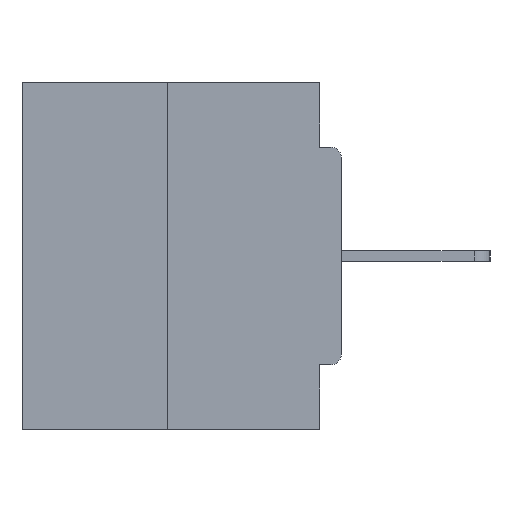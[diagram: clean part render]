
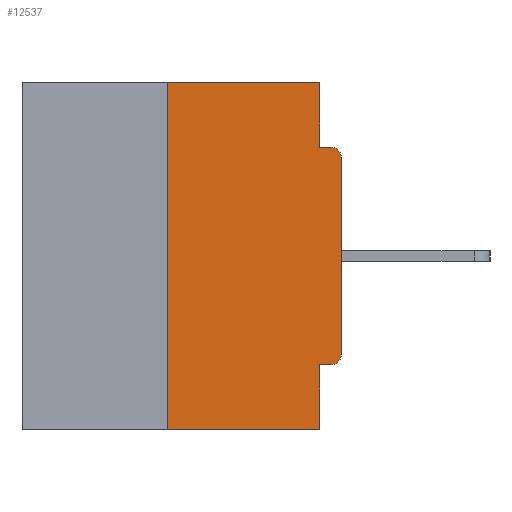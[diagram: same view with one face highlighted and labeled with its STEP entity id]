
A CAD part, left-side view. The second image highlights one B-rep face of the part: STEP entity #12537.
In plain terms, the highlighted planar face has unit normal (-1, 0, 0).
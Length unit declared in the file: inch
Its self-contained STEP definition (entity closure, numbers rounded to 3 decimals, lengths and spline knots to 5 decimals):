
#503 = DIRECTION ( 'NONE',  ( 0., 0., -1. ) ) ;
#929 = ORIENTED_EDGE ( 'NONE', *, *, #15177, .T. ) ;
#1581 = CARTESIAN_POINT ( 'NONE',  ( 0., 0.015, -0.4065 ) ) ;
#2330 = PLANE ( 'NONE',  #23668 ) ;
#2412 = VERTEX_POINT ( 'NONE', #6852 ) ;
#2626 = FACE_OUTER_BOUND ( 'NONE', #9411, .T. ) ;
#2676 = DIRECTION ( 'NONE',  ( 0., -1., 0. ) ) ;
#3253 = VECTOR ( 'NONE', #3336, 39.37008 ) ;
#3336 = DIRECTION ( 'NONE',  ( 0., 0., 1. ) ) ;
#3755 = DIRECTION ( 'NONE',  ( 0., 1., 0. ) ) ;
#4030 = LINE ( 'NONE', #31475, #20502 ) ;
#4177 = CARTESIAN_POINT ( 'NONE',  ( 0., 0.031, -0.5 ) ) ;
#4433 = LINE ( 'NONE', #6392, #27638 ) ;
#5618 = CARTESIAN_POINT ( 'NONE',  ( 0., 0.015, -0.3915 ) ) ;
#5665 = VERTEX_POINT ( 'NONE', #16105 ) ;
#6120 = LINE ( 'NONE', #13108, #3253 ) ;
#6241 = ORIENTED_EDGE ( 'NONE', *, *, #26397, .F. ) ;
#6304 = CARTESIAN_POINT ( 'NONE',  ( 0., 0.25, -0.5 ) ) ;
#6392 = CARTESIAN_POINT ( 'NONE',  ( 0., 0.25, 0. ) ) ;
#6852 = CARTESIAN_POINT ( 'NONE',  ( 0., 0.25, 0. ) ) ;
#7880 = VERTEX_POINT ( 'NONE', #9330 ) ;
#8070 = CARTESIAN_POINT ( 'NONE',  ( 0., 0., -0.4065 ) ) ;
#8222 = ORIENTED_EDGE ( 'NONE', *, *, #12829, .F. ) ;
#8256 = CARTESIAN_POINT ( 'NONE',  ( 0., 0.031, -0.0935 ) ) ;
#8479 = DIRECTION ( 'NONE',  ( 0., -1., 0. ) ) ;
#9048 = CARTESIAN_POINT ( 'NONE',  ( 0., 0.015, -0.1085 ) ) ;
#9330 = CARTESIAN_POINT ( 'NONE',  ( 0., 0.031, -0.4065 ) ) ;
#9411 = EDGE_LOOP ( 'NONE', ( #23773, #20358, #26169, #8222, #23984, #16713, #929, #14431, #6241, #16101 ) ) ;
#9448 = VERTEX_POINT ( 'NONE', #8256 ) ;
#9964 = EDGE_CURVE ( 'NONE', #26094, #10788, #29596, .T. ) ;
#10181 = DIRECTION ( 'NONE',  ( -1., 0., 0. ) ) ;
#10189 = LINE ( 'NONE', #24910, #29163 ) ;
#10788 = VERTEX_POINT ( 'NONE', #4177 ) ;
#11238 = EDGE_CURVE ( 'NONE', #30255, #18971, #11593, .T. ) ;
#11593 = CIRCLE ( 'NONE', #17828, 0.015 ) ;
#11639 = DIRECTION ( 'NONE',  ( 0., -1., 0. ) ) ;
#12537 = ADVANCED_FACE ( 'NONE', ( #2626 ), #2330, .F. ) ;
#12764 = CARTESIAN_POINT ( 'NONE',  ( 0., 0.031, 0. ) ) ;
#12829 = EDGE_CURVE ( 'NONE', #7880, #10788, #31689, .T. ) ;
#13108 = CARTESIAN_POINT ( 'NONE',  ( 0., 0., 0. ) ) ;
#13932 = EDGE_CURVE ( 'NONE', #21062, #7880, #16162, .T. ) ;
#14431 = ORIENTED_EDGE ( 'NONE', *, *, #11238, .T. ) ;
#15177 = EDGE_CURVE ( 'NONE', #5665, #30255, #6120, .T. ) ;
#15244 = VECTOR ( 'NONE', #23862, 39.37008 ) ;
#15352 = VECTOR ( 'NONE', #8479, 39.37008 ) ;
#15406 = CARTESIAN_POINT ( 'NONE',  ( 0., 0., -0.1085 ) ) ;
#15830 = LINE ( 'NONE', #23199, #15352 ) ;
#16101 = ORIENTED_EDGE ( 'NONE', *, *, #21096, .F. ) ;
#16105 = CARTESIAN_POINT ( 'NONE',  ( 0., 0., -0.3915 ) ) ;
#16162 = LINE ( 'NONE', #8070, #16819 ) ;
#16713 = ORIENTED_EDGE ( 'NONE', *, *, #30251, .T. ) ;
#16736 = DIRECTION ( 'NONE',  ( 0., 0., -1. ) ) ;
#16819 = VECTOR ( 'NONE', #3755, 39.37008 ) ;
#17487 = DIRECTION ( 'NONE',  ( 1., 0., 0. ) ) ;
#17828 = AXIS2_PLACEMENT_3D ( 'NONE', #9048, #22105, #26863 ) ;
#18017 = DIRECTION ( 'NONE',  ( 0., 0., -1. ) ) ;
#18971 = VERTEX_POINT ( 'NONE', #28110 ) ;
#19381 = AXIS2_PLACEMENT_3D ( 'NONE', #5618, #10181, #18017 ) ;
#20358 = ORIENTED_EDGE ( 'NONE', *, *, #27040, .F. ) ;
#20502 = VECTOR ( 'NONE', #16736, 39.37008 ) ;
#21062 = VERTEX_POINT ( 'NONE', #1581 ) ;
#21096 = EDGE_CURVE ( 'NONE', #21788, #9448, #4030, .T. ) ;
#21788 = VERTEX_POINT ( 'NONE', #12764 ) ;
#21997 = CIRCLE ( 'NONE', #19381, 0.015 ) ;
#22105 = DIRECTION ( 'NONE',  ( -1., 0., 0. ) ) ;
#22332 = EDGE_CURVE ( 'NONE', #2412, #21788, #15830, .T. ) ;
#23199 = CARTESIAN_POINT ( 'NONE',  ( 0., 0.46, 0. ) ) ;
#23668 = AXIS2_PLACEMENT_3D ( 'NONE', #27617, #17487, #503 ) ;
#23773 = ORIENTED_EDGE ( 'NONE', *, *, #22332, .F. ) ;
#23862 = DIRECTION ( 'NONE',  ( 0., 0., -1. ) ) ;
#23984 = ORIENTED_EDGE ( 'NONE', *, *, #13932, .F. ) ;
#24233 = CARTESIAN_POINT ( 'NONE',  ( 0., 0.46, -0.5 ) ) ;
#24910 = CARTESIAN_POINT ( 'NONE',  ( 0., 0., -0.0935 ) ) ;
#26094 = VERTEX_POINT ( 'NONE', #6304 ) ;
#26169 = ORIENTED_EDGE ( 'NONE', *, *, #9964, .T. ) ;
#26397 = EDGE_CURVE ( 'NONE', #9448, #18971, #10189, .T. ) ;
#26863 = DIRECTION ( 'NONE',  ( 0., 0., -1. ) ) ;
#27040 = EDGE_CURVE ( 'NONE', #26094, #2412, #4433, .T. ) ;
#27617 = CARTESIAN_POINT ( 'NONE',  ( 0., 0.46, 0. ) ) ;
#27638 = VECTOR ( 'NONE', #29415, 39.37008 ) ;
#28110 = CARTESIAN_POINT ( 'NONE',  ( 0., 0.015, -0.0935 ) ) ;
#28922 = CARTESIAN_POINT ( 'NONE',  ( 0., 0.031, -0.5 ) ) ;
#29163 = VECTOR ( 'NONE', #2676, 39.37008 ) ;
#29415 = DIRECTION ( 'NONE',  ( 0., 0., 1. ) ) ;
#29596 = LINE ( 'NONE', #24233, #32268 ) ;
#30251 = EDGE_CURVE ( 'NONE', #21062, #5665, #21997, .T. ) ;
#30255 = VERTEX_POINT ( 'NONE', #15406 ) ;
#31475 = CARTESIAN_POINT ( 'NONE',  ( 0., 0.031, 0. ) ) ;
#31689 = LINE ( 'NONE', #28922, #15244 ) ;
#32268 = VECTOR ( 'NONE', #11639, 39.37008 ) ;
